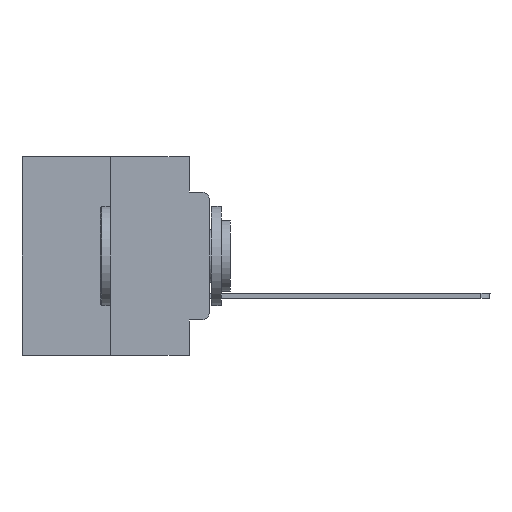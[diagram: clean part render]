
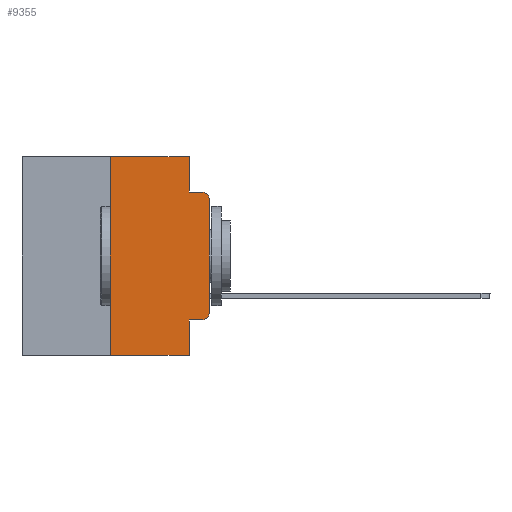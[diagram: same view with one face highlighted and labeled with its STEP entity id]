
A CAD part, left-side view. The second image highlights one B-rep face of the part: STEP entity #9355.
In plain terms, the highlighted planar face has unit normal (-1, 0, 0).
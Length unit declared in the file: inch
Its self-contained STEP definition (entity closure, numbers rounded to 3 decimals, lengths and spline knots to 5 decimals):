
#437 = ORIENTED_EDGE ( 'NONE', *, *, #3985, .F. ) ;
#877 = CARTESIAN_POINT ( 'NONE',  ( 0., 0.02, -0.4115 ) ) ;
#1177 = CARTESIAN_POINT ( 'NONE',  ( 0., 0.051, 0. ) ) ;
#1848 = VERTEX_POINT ( 'NONE', #877 ) ;
#2355 = CIRCLE ( 'NONE', #21827, 0.02 ) ;
#2405 = ORIENTED_EDGE ( 'NONE', *, *, #9829, .T. ) ;
#2638 = LINE ( 'NONE', #23350, #5439 ) ;
#2771 = DIRECTION ( 'NONE',  ( 0., -1., 0. ) ) ;
#3313 = ORIENTED_EDGE ( 'NONE', *, *, #26472, .F. ) ;
#3362 = EDGE_CURVE ( 'NONE', #14865, #25532, #17679, .T. ) ;
#3820 = DIRECTION ( 'NONE',  ( 0., -1., 0. ) ) ;
#3943 = EDGE_CURVE ( 'NONE', #9403, #7567, #8156, .T. ) ;
#3985 = EDGE_CURVE ( 'NONE', #5860, #14865, #22188, .T. ) ;
#4159 = VERTEX_POINT ( 'NONE', #9554 ) ;
#4231 = DIRECTION ( 'NONE',  ( -1., 0., 0. ) ) ;
#5316 = LINE ( 'NONE', #20334, #17755 ) ;
#5439 = VECTOR ( 'NONE', #2771, 39.37008 ) ;
#5544 = CARTESIAN_POINT ( 'NONE',  ( 0., 0.25, 0. ) ) ;
#5679 = DIRECTION ( 'NONE',  ( 0., 0., 1. ) ) ;
#5801 = ORIENTED_EDGE ( 'NONE', *, *, #10535, .T. ) ;
#5860 = VERTEX_POINT ( 'NONE', #25377 ) ;
#6128 = CARTESIAN_POINT ( 'NONE',  ( 0., 0.02, -0.0885 ) ) ;
#6266 = CARTESIAN_POINT ( 'NONE',  ( 0., 0.02, -0.3915 ) ) ;
#6404 = EDGE_LOOP ( 'NONE', ( #9325, #21908, #25774, #3313, #20287, #437, #2405, #12818, #5801, #7099 ) ) ;
#6481 = CARTESIAN_POINT ( 'NONE',  ( 0., 0., -0.3915 ) ) ;
#6657 = VECTOR ( 'NONE', #24296, 39.37008 ) ;
#6969 = CARTESIAN_POINT ( 'NONE',  ( 0., 0., -0.1085 ) ) ;
#7099 = ORIENTED_EDGE ( 'NONE', *, *, #22771, .T. ) ;
#7170 = VECTOR ( 'NONE', #5679, 39.37008 ) ;
#7547 = LINE ( 'NONE', #1177, #17904 ) ;
#7567 = VERTEX_POINT ( 'NONE', #9501 ) ;
#7825 = CARTESIAN_POINT ( 'NONE',  ( 0., 0.25, 0. ) ) ;
#8156 = LINE ( 'NONE', #18592, #9324 ) ;
#8286 = DIRECTION ( 'NONE',  ( 0., 0., -1. ) ) ;
#8320 = DIRECTION ( 'NONE',  ( 0., 0., -1. ) ) ;
#9276 = DIRECTION ( 'NONE',  ( 0., 0., -1. ) ) ;
#9311 = VERTEX_POINT ( 'NONE', #6481 ) ;
#9324 = VECTOR ( 'NONE', #8286, 39.37008 ) ;
#9325 = ORIENTED_EDGE ( 'NONE', *, *, #22559, .T. ) ;
#9355 = ADVANCED_FACE ( 'NONE', ( #14740 ), #18947, .F. ) ;
#9403 = VERTEX_POINT ( 'NONE', #17695 ) ;
#9501 = CARTESIAN_POINT ( 'NONE',  ( 0., 0.051, -0.5 ) ) ;
#9554 = CARTESIAN_POINT ( 'NONE',  ( 0., 0.051, -0.0885 ) ) ;
#9782 = CARTESIAN_POINT ( 'NONE',  ( 0., 0.051, 0. ) ) ;
#9829 = EDGE_CURVE ( 'NONE', #5860, #7567, #2638, .T. ) ;
#9975 = EDGE_CURVE ( 'NONE', #17782, #22586, #12972, .T. ) ;
#10535 = EDGE_CURVE ( 'NONE', #9403, #1848, #5316, .T. ) ;
#11282 = VECTOR ( 'NONE', #18835, 39.37008 ) ;
#12818 = ORIENTED_EDGE ( 'NONE', *, *, #3943, .F. ) ;
#12972 = CIRCLE ( 'NONE', #18161, 0.02 ) ;
#12991 = LINE ( 'NONE', #20721, #11282 ) ;
#13620 = VECTOR ( 'NONE', #16424, 39.37008 ) ;
#14740 = FACE_OUTER_BOUND ( 'NONE', #6404, .T. ) ;
#14865 = VERTEX_POINT ( 'NONE', #7825 ) ;
#16424 = DIRECTION ( 'NONE',  ( 0., 0., 1. ) ) ;
#17679 = LINE ( 'NONE', #25791, #6657 ) ;
#17695 = CARTESIAN_POINT ( 'NONE',  ( 0., 0.051, -0.4115 ) ) ;
#17755 = VECTOR ( 'NONE', #3820, 39.37008 ) ;
#17782 = VERTEX_POINT ( 'NONE', #6969 ) ;
#17904 = VECTOR ( 'NONE', #8320, 39.37008 ) ;
#18032 = AXIS2_PLACEMENT_3D ( 'NONE', #23107, #24740, #22971 ) ;
#18161 = AXIS2_PLACEMENT_3D ( 'NONE', #19572, #25780, #9276 ) ;
#18592 = CARTESIAN_POINT ( 'NONE',  ( 0., 0.051, 0. ) ) ;
#18736 = EDGE_CURVE ( 'NONE', #4159, #22586, #12991, .T. ) ;
#18835 = DIRECTION ( 'NONE',  ( 0., -1., 0. ) ) ;
#18947 = PLANE ( 'NONE',  #18032 ) ;
#19572 = CARTESIAN_POINT ( 'NONE',  ( 0., 0.02, -0.1085 ) ) ;
#20219 = LINE ( 'NONE', #26562, #13620 ) ;
#20287 = ORIENTED_EDGE ( 'NONE', *, *, #3362, .F. ) ;
#20334 = CARTESIAN_POINT ( 'NONE',  ( 0., 0.051, -0.4115 ) ) ;
#20721 = CARTESIAN_POINT ( 'NONE',  ( 0., 0.051, -0.0885 ) ) ;
#21827 = AXIS2_PLACEMENT_3D ( 'NONE', #6266, #4231, #25990 ) ;
#21908 = ORIENTED_EDGE ( 'NONE', *, *, #9975, .T. ) ;
#22188 = LINE ( 'NONE', #5544, #7170 ) ;
#22559 = EDGE_CURVE ( 'NONE', #9311, #17782, #20219, .T. ) ;
#22586 = VERTEX_POINT ( 'NONE', #6128 ) ;
#22771 = EDGE_CURVE ( 'NONE', #1848, #9311, #2355, .T. ) ;
#22971 = DIRECTION ( 'NONE',  ( 0., 0., -1. ) ) ;
#23107 = CARTESIAN_POINT ( 'NONE',  ( 0., 0.473, 0. ) ) ;
#23350 = CARTESIAN_POINT ( 'NONE',  ( 0., 0.473, -0.5 ) ) ;
#24296 = DIRECTION ( 'NONE',  ( 0., -1., 0. ) ) ;
#24740 = DIRECTION ( 'NONE',  ( 1., 0., 0. ) ) ;
#25377 = CARTESIAN_POINT ( 'NONE',  ( 0., 0.25, -0.5 ) ) ;
#25532 = VERTEX_POINT ( 'NONE', #9782 ) ;
#25774 = ORIENTED_EDGE ( 'NONE', *, *, #18736, .F. ) ;
#25780 = DIRECTION ( 'NONE',  ( -1., 0., 0. ) ) ;
#25791 = CARTESIAN_POINT ( 'NONE',  ( 0., 0.473, 0. ) ) ;
#25990 = DIRECTION ( 'NONE',  ( 0., 0., -1. ) ) ;
#26472 = EDGE_CURVE ( 'NONE', #25532, #4159, #7547, .T. ) ;
#26562 = CARTESIAN_POINT ( 'NONE',  ( 0., 0., 0. ) ) ;
